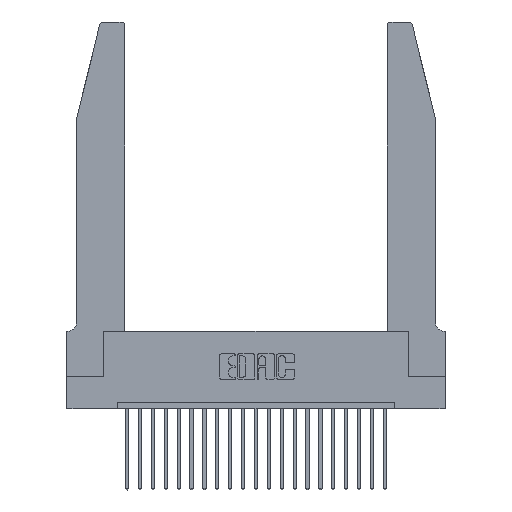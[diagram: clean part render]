
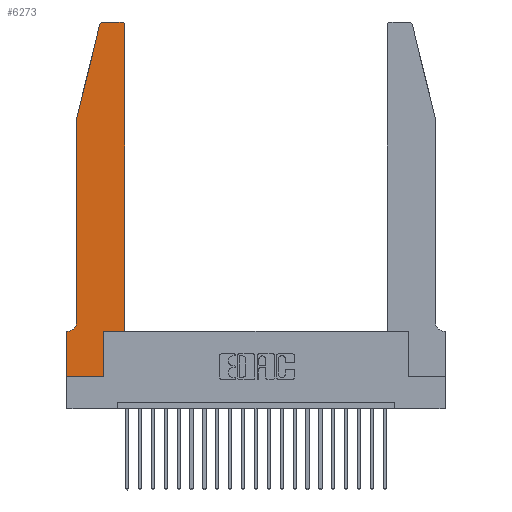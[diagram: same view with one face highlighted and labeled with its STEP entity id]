
A CAD part, top view. The second image highlights one B-rep face of the part: STEP entity #6273.
In plain terms, the highlighted planar face has unit normal (0, 0, 1).
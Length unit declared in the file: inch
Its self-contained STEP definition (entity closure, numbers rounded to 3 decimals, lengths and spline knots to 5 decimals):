
#420 = DIRECTION ( 'NONE',  ( 1., 0., 0. ) ) ;
#426 = CARTESIAN_POINT ( 'NONE',  ( 0.2605, 2.75, 0.37 ) ) ;
#551 = LINE ( 'NONE', #4924, #11841 ) ;
#552 = ORIENTED_EDGE ( 'NONE', *, *, #4148, .T. ) ;
#755 = VERTEX_POINT ( 'NONE', #19033 ) ;
#1202 = VECTOR ( 'NONE', #17489, 39.37008 ) ;
#1260 = CARTESIAN_POINT ( 'NONE',  ( 0.0055, 0.35, 0.37 ) ) ;
#1338 = DIRECTION ( 'NONE',  ( 1., 0., 0. ) ) ;
#1378 = EDGE_CURVE ( 'NONE', #15948, #8648, #22944, .T. ) ;
#1667 = DIRECTION ( 'NONE',  ( 1., 0., 0. ) ) ;
#1873 = VECTOR ( 'NONE', #420, 39.37008 ) ;
#1901 = ORIENTED_EDGE ( 'NONE', *, *, #22368, .T. ) ;
#3288 = LINE ( 'NONE', #5834, #1873 ) ;
#3533 = CARTESIAN_POINT ( 'NONE',  ( 0.0755, 2., 0.37 ) ) ;
#3899 = LINE ( 'NONE', #11020, #19150 ) ;
#4148 = EDGE_CURVE ( 'NONE', #10409, #18342, #3899, .T. ) ;
#4405 = EDGE_CURVE ( 'NONE', #16236, #7851, #9543, .T. ) ;
#4924 = CARTESIAN_POINT ( 'NONE',  ( 0.2865, 0.35, 0.37 ) ) ;
#5312 = DIRECTION ( 'NONE',  ( -1., 0., 0. ) ) ;
#5362 = CIRCLE ( 'NONE', #16506, 0.03 ) ;
#5423 = CIRCLE ( 'NONE', #22379, 0.03 ) ;
#5834 = CARTESIAN_POINT ( 'NONE',  ( 0., 0., 0.37 ) ) ;
#6050 = LINE ( 'NONE', #13862, #1202 ) ;
#6273 = ADVANCED_FACE ( 'NONE', ( #10309 ), #7400, .T. ) ;
#6800 = VERTEX_POINT ( 'NONE', #12736 ) ;
#6960 = EDGE_CURVE ( 'NONE', #7851, #10409, #6050, .T. ) ;
#6984 = CARTESIAN_POINT ( 'NONE',  ( 0., 0.35, 0.37 ) ) ;
#7075 = DIRECTION ( 'NONE',  ( 0., 0., 1. ) ) ;
#7314 = DIRECTION ( 'NONE',  ( -0.239, -0.971, 0. ) ) ;
#7400 = PLANE ( 'NONE',  #20225 ) ;
#7651 = EDGE_CURVE ( 'NONE', #16069, #8868, #5423, .T. ) ;
#7851 = VERTEX_POINT ( 'NONE', #1260 ) ;
#8032 = EDGE_CURVE ( 'NONE', #22866, #6800, #9914, .T. ) ;
#8556 = DIRECTION ( 'NONE',  ( 0., 1., 0. ) ) ;
#8642 = EDGE_CURVE ( 'NONE', #755, #22866, #551, .T. ) ;
#8648 = VERTEX_POINT ( 'NONE', #10189 ) ;
#8702 = VERTEX_POINT ( 'NONE', #23431 ) ;
#8751 = CARTESIAN_POINT ( 'NONE',  ( 0.4505, 2.72, 0.37 ) ) ;
#8806 = EDGE_CURVE ( 'NONE', #8868, #8702, #16637, .T. ) ;
#8868 = VERTEX_POINT ( 'NONE', #20155 ) ;
#9029 = CARTESIAN_POINT ( 'NONE',  ( 0.284, 2.72, 0.37 ) ) ;
#9143 = DIRECTION ( 'NONE',  ( 0., -1., 0. ) ) ;
#9357 = ORIENTED_EDGE ( 'NONE', *, *, #8032, .T. ) ;
#9543 = CIRCLE ( 'NONE', #15660, 0.07 ) ;
#9914 = LINE ( 'NONE', #17071, #17502 ) ;
#9949 = CARTESIAN_POINT ( 'NONE',  ( 0.0755, 0.42, 0.37 ) ) ;
#10189 = CARTESIAN_POINT ( 'NONE',  ( 0.0755, 2., 0.37 ) ) ;
#10309 = FACE_OUTER_BOUND ( 'NONE', #10890, .T. ) ;
#10409 = VERTEX_POINT ( 'NONE', #6984 ) ;
#10890 = EDGE_LOOP ( 'NONE', ( #17946, #1901, #18098, #13785, #22422, #18024, #552, #11441, #14487, #9357, #20946, #14117 ) ) ;
#11011 = DIRECTION ( 'NONE',  ( 0., 0., 1. ) ) ;
#11020 = CARTESIAN_POINT ( 'NONE',  ( 0., 0., 0.37 ) ) ;
#11241 = DIRECTION ( 'NONE',  ( 0., 1., 0. ) ) ;
#11441 = ORIENTED_EDGE ( 'NONE', *, *, #17724, .T. ) ;
#11841 = VECTOR ( 'NONE', #8556, 39.37008 ) ;
#12049 = CARTESIAN_POINT ( 'NONE',  ( 0.4205, 2.72, 0.37 ) ) ;
#12736 = CARTESIAN_POINT ( 'NONE',  ( 0.4505, 0.35, 0.37 ) ) ;
#13055 = CARTESIAN_POINT ( 'NONE',  ( 0.2865, 0.35, 0.37 ) ) ;
#13107 = VECTOR ( 'NONE', #13223, 39.37008 ) ;
#13223 = DIRECTION ( 'NONE',  ( 0., -1., 0. ) ) ;
#13785 = ORIENTED_EDGE ( 'NONE', *, *, #19241, .T. ) ;
#13862 = CARTESIAN_POINT ( 'NONE',  ( 0.0755, 0.35, 0.37 ) ) ;
#14117 = ORIENTED_EDGE ( 'NONE', *, *, #7651, .T. ) ;
#14223 = LINE ( 'NONE', #3533, #13107 ) ;
#14487 = ORIENTED_EDGE ( 'NONE', *, *, #8642, .T. ) ;
#15660 = AXIS2_PLACEMENT_3D ( 'NONE', #18185, #20017, #5312 ) ;
#15948 = VERTEX_POINT ( 'NONE', #20010 ) ;
#15950 = DIRECTION ( 'NONE',  ( 1., 0., 0. ) ) ;
#16069 = VERTEX_POINT ( 'NONE', #8751 ) ;
#16236 = VERTEX_POINT ( 'NONE', #9949 ) ;
#16315 = VECTOR ( 'NONE', #11241, 39.37008 ) ;
#16348 = CARTESIAN_POINT ( 'NONE',  ( 0.4505, 0.35, 0.37 ) ) ;
#16441 = EDGE_CURVE ( 'NONE', #6800, #16069, #17171, .T. ) ;
#16506 = AXIS2_PLACEMENT_3D ( 'NONE', #9029, #7075, #1667 ) ;
#16637 = LINE ( 'NONE', #426, #20886 ) ;
#17071 = CARTESIAN_POINT ( 'NONE',  ( 0.4505, 0.35, 0.37 ) ) ;
#17171 = LINE ( 'NONE', #16348, #16315 ) ;
#17251 = VECTOR ( 'NONE', #7314, 39.37008 ) ;
#17484 = DIRECTION ( 'NONE',  ( 0., 0., 1. ) ) ;
#17489 = DIRECTION ( 'NONE',  ( -1., 0., 0. ) ) ;
#17502 = VECTOR ( 'NONE', #15950, 39.37008 ) ;
#17724 = EDGE_CURVE ( 'NONE', #18342, #755, #3288, .T. ) ;
#17946 = ORIENTED_EDGE ( 'NONE', *, *, #8806, .T. ) ;
#18024 = ORIENTED_EDGE ( 'NONE', *, *, #6960, .T. ) ;
#18081 = CARTESIAN_POINT ( 'NONE',  ( 0.0755, 2., 0.37 ) ) ;
#18098 = ORIENTED_EDGE ( 'NONE', *, *, #1378, .T. ) ;
#18185 = CARTESIAN_POINT ( 'NONE',  ( 0.0055, 0.42, 0.37 ) ) ;
#18342 = VERTEX_POINT ( 'NONE', #19720 ) ;
#19033 = CARTESIAN_POINT ( 'NONE',  ( 0.2865, 0., 0.37 ) ) ;
#19150 = VECTOR ( 'NONE', #9143, 39.37008 ) ;
#19241 = EDGE_CURVE ( 'NONE', #8648, #16236, #14223, .T. ) ;
#19720 = CARTESIAN_POINT ( 'NONE',  ( 0., 0., 0.37 ) ) ;
#20010 = CARTESIAN_POINT ( 'NONE',  ( 0.25487, 2.72718, 0.37 ) ) ;
#20017 = DIRECTION ( 'NONE',  ( 0., 0., -1. ) ) ;
#20091 = DIRECTION ( 'NONE',  ( 1., 0., 0. ) ) ;
#20155 = CARTESIAN_POINT ( 'NONE',  ( 0.4205, 2.75, 0.37 ) ) ;
#20225 = AXIS2_PLACEMENT_3D ( 'NONE', #21817, #11011, #20091 ) ;
#20886 = VECTOR ( 'NONE', #22145, 39.37008 ) ;
#20946 = ORIENTED_EDGE ( 'NONE', *, *, #16441, .T. ) ;
#21817 = CARTESIAN_POINT ( 'NONE',  ( 0., 0.35, 0.37 ) ) ;
#22145 = DIRECTION ( 'NONE',  ( -1., 0., 0. ) ) ;
#22368 = EDGE_CURVE ( 'NONE', #8702, #15948, #5362, .T. ) ;
#22379 = AXIS2_PLACEMENT_3D ( 'NONE', #12049, #17484, #1338 ) ;
#22422 = ORIENTED_EDGE ( 'NONE', *, *, #4405, .T. ) ;
#22866 = VERTEX_POINT ( 'NONE', #13055 ) ;
#22944 = LINE ( 'NONE', #18081, #17251 ) ;
#23431 = CARTESIAN_POINT ( 'NONE',  ( 0.284, 2.75, 0.37 ) ) ;
